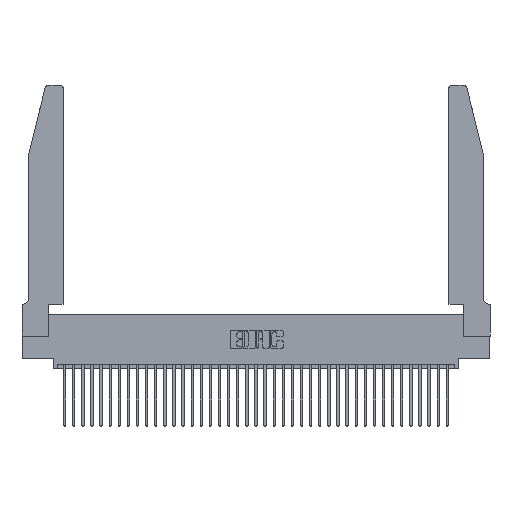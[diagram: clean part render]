
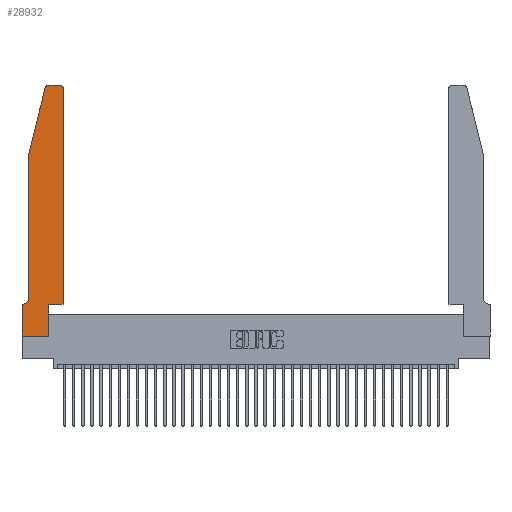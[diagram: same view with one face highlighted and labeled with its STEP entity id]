
A CAD part, top view. The second image highlights one B-rep face of the part: STEP entity #28932.
In plain terms, the highlighted planar face has unit normal (0, 0, 1).
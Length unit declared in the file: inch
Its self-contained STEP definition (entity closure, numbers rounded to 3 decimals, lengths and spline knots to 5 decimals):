
#304 = VERTEX_POINT ( 'NONE', #25919 ) ;
#470 = DIRECTION ( 'NONE',  ( 0., -1., 0. ) ) ;
#1260 = CARTESIAN_POINT ( 'NONE',  ( 0.2605, 2.75, 0.37 ) ) ;
#1505 = EDGE_CURVE ( 'NONE', #33175, #14785, #15760, .T. ) ;
#1660 = DIRECTION ( 'NONE',  ( -1., 0., 0. ) ) ;
#2172 = CARTESIAN_POINT ( 'NONE',  ( 0.4505, 2.72, 0.37 ) ) ;
#2261 = CIRCLE ( 'NONE', #24599, 0.07 ) ;
#3043 = LINE ( 'NONE', #6097, #34599 ) ;
#3149 = ORIENTED_EDGE ( 'NONE', *, *, #13100, .T. ) ;
#3278 = LINE ( 'NONE', #36881, #11348 ) ;
#3804 = CARTESIAN_POINT ( 'NONE',  ( 0.284, 2.72, 0.37 ) ) ;
#3981 = EDGE_CURVE ( 'NONE', #18993, #304, #12584, .T. ) ;
#4358 = DIRECTION ( 'NONE',  ( -1., 0., 0. ) ) ;
#4761 = EDGE_CURVE ( 'NONE', #7552, #15856, #3043, .T. ) ;
#4912 = CARTESIAN_POINT ( 'NONE',  ( 0.0755, 0.42, 0.37 ) ) ;
#4940 = EDGE_CURVE ( 'NONE', #19021, #33175, #29123, .T. ) ;
#5547 = ORIENTED_EDGE ( 'NONE', *, *, #11394, .T. ) ;
#6097 = CARTESIAN_POINT ( 'NONE',  ( 0., 0., 0.37 ) ) ;
#6327 = LINE ( 'NONE', #34366, #13416 ) ;
#6595 = LINE ( 'NONE', #31458, #21521 ) ;
#6859 = DIRECTION ( 'NONE',  ( 1., 0., 0. ) ) ;
#7552 = VERTEX_POINT ( 'NONE', #10192 ) ;
#7788 = AXIS2_PLACEMENT_3D ( 'NONE', #24036, #35851, #18290 ) ;
#7964 = CARTESIAN_POINT ( 'NONE',  ( 0.25487, 2.72718, 0.37 ) ) ;
#8572 = VERTEX_POINT ( 'NONE', #38523 ) ;
#9443 = CARTESIAN_POINT ( 'NONE',  ( 0.4505, 0.35, 0.37 ) ) ;
#10177 = DIRECTION ( 'NONE',  ( 1., 0., 0. ) ) ;
#10192 = CARTESIAN_POINT ( 'NONE',  ( 0., 0.35, 0.37 ) ) ;
#10403 = VECTOR ( 'NONE', #24217, 39.37008 ) ;
#11271 = ORIENTED_EDGE ( 'NONE', *, *, #35568, .T. ) ;
#11348 = VECTOR ( 'NONE', #13345, 39.37008 ) ;
#11394 = EDGE_CURVE ( 'NONE', #8572, #18993, #33924, .T. ) ;
#11658 = ORIENTED_EDGE ( 'NONE', *, *, #33771, .T. ) ;
#12418 = FACE_OUTER_BOUND ( 'NONE', #30253, .T. ) ;
#12584 = CIRCLE ( 'NONE', #25155, 0.03 ) ;
#13100 = EDGE_CURVE ( 'NONE', #26247, #27974, #2261, .T. ) ;
#13345 = DIRECTION ( 'NONE',  ( -1., 0., 0. ) ) ;
#13416 = VECTOR ( 'NONE', #28503, 39.37008 ) ;
#13908 = VECTOR ( 'NONE', #35479, 39.37008 ) ;
#14070 = ORIENTED_EDGE ( 'NONE', *, *, #4940, .T. ) ;
#14584 = CARTESIAN_POINT ( 'NONE',  ( 0.4205, 2.72, 0.37 ) ) ;
#14785 = VERTEX_POINT ( 'NONE', #27645 ) ;
#15078 = AXIS2_PLACEMENT_3D ( 'NONE', #3804, #24675, #6859 ) ;
#15760 = LINE ( 'NONE', #38482, #13908 ) ;
#15856 = VERTEX_POINT ( 'NONE', #31066 ) ;
#15868 = VECTOR ( 'NONE', #470, 39.37008 ) ;
#16857 = DIRECTION ( 'NONE',  ( 1., 0., 0. ) ) ;
#17361 = CARTESIAN_POINT ( 'NONE',  ( 0.284, 2.75, 0.37 ) ) ;
#17573 = DIRECTION ( 'NONE',  ( 1., 0., 0. ) ) ;
#18290 = DIRECTION ( 'NONE',  ( 1., 0., 0. ) ) ;
#18993 = VERTEX_POINT ( 'NONE', #2172 ) ;
#19021 = VERTEX_POINT ( 'NONE', #17361 ) ;
#19700 = DIRECTION ( 'NONE',  ( 0., 0., -1. ) ) ;
#20292 = VERTEX_POINT ( 'NONE', #37680 ) ;
#20692 = VECTOR ( 'NONE', #10177, 39.37008 ) ;
#21521 = VECTOR ( 'NONE', #16857, 39.37008 ) ;
#22002 = CARTESIAN_POINT ( 'NONE',  ( 0., 0., 0.37 ) ) ;
#22232 = ORIENTED_EDGE ( 'NONE', *, *, #3981, .T. ) ;
#22586 = ORIENTED_EDGE ( 'NONE', *, *, #33668, .T. ) ;
#23254 = EDGE_CURVE ( 'NONE', #15856, #20292, #28497, .T. ) ;
#23681 = LINE ( 'NONE', #33263, #15868 ) ;
#23896 = DIRECTION ( 'NONE',  ( 0., -1., 0. ) ) ;
#24036 = CARTESIAN_POINT ( 'NONE',  ( 0., 0.35, 0.37 ) ) ;
#24217 = DIRECTION ( 'NONE',  ( 0., 1., 0. ) ) ;
#24599 = AXIS2_PLACEMENT_3D ( 'NONE', #37275, #19700, #1660 ) ;
#24671 = VECTOR ( 'NONE', #4358, 39.37008 ) ;
#24675 = DIRECTION ( 'NONE',  ( 0., 0., 1. ) ) ;
#25155 = AXIS2_PLACEMENT_3D ( 'NONE', #14584, #35128, #17573 ) ;
#25919 = CARTESIAN_POINT ( 'NONE',  ( 0.4205, 2.75, 0.37 ) ) ;
#26247 = VERTEX_POINT ( 'NONE', #4912 ) ;
#27224 = ORIENTED_EDGE ( 'NONE', *, *, #23254, .T. ) ;
#27645 = CARTESIAN_POINT ( 'NONE',  ( 0.0755, 2., 0.37 ) ) ;
#27974 = VERTEX_POINT ( 'NONE', #33957 ) ;
#28497 = LINE ( 'NONE', #22002, #20692 ) ;
#28503 = DIRECTION ( 'NONE',  ( 0., 1., 0. ) ) ;
#28932 = ADVANCED_FACE ( 'NONE', ( #12418 ), #32881, .T. ) ;
#29004 = EDGE_CURVE ( 'NONE', #14785, #26247, #23681, .T. ) ;
#29123 = CIRCLE ( 'NONE', #15078, 0.03 ) ;
#30253 = EDGE_LOOP ( 'NONE', ( #11271, #14070, #34969, #38028, #3149, #22586, #33823, #27224, #36115, #11658, #5547, #22232 ) ) ;
#30467 = CARTESIAN_POINT ( 'NONE',  ( 0.2865, 0.35, 0.37 ) ) ;
#31066 = CARTESIAN_POINT ( 'NONE',  ( 0., 0., 0.37 ) ) ;
#31351 = EDGE_CURVE ( 'NONE', #20292, #34916, #6327, .T. ) ;
#31458 = CARTESIAN_POINT ( 'NONE',  ( 0.4505, 0.35, 0.37 ) ) ;
#32881 = PLANE ( 'NONE',  #7788 ) ;
#33175 = VERTEX_POINT ( 'NONE', #7964 ) ;
#33263 = CARTESIAN_POINT ( 'NONE',  ( 0.0755, 2., 0.37 ) ) ;
#33372 = LINE ( 'NONE', #1260, #24671 ) ;
#33668 = EDGE_CURVE ( 'NONE', #27974, #7552, #3278, .T. ) ;
#33771 = EDGE_CURVE ( 'NONE', #34916, #8572, #6595, .T. ) ;
#33823 = ORIENTED_EDGE ( 'NONE', *, *, #4761, .T. ) ;
#33924 = LINE ( 'NONE', #9443, #10403 ) ;
#33957 = CARTESIAN_POINT ( 'NONE',  ( 0.0055, 0.35, 0.37 ) ) ;
#34366 = CARTESIAN_POINT ( 'NONE',  ( 0.2865, 0.35, 0.37 ) ) ;
#34599 = VECTOR ( 'NONE', #23896, 39.37008 ) ;
#34916 = VERTEX_POINT ( 'NONE', #30467 ) ;
#34969 = ORIENTED_EDGE ( 'NONE', *, *, #1505, .T. ) ;
#35128 = DIRECTION ( 'NONE',  ( 0., 0., 1. ) ) ;
#35479 = DIRECTION ( 'NONE',  ( -0.239, -0.971, 0. ) ) ;
#35568 = EDGE_CURVE ( 'NONE', #304, #19021, #33372, .T. ) ;
#35851 = DIRECTION ( 'NONE',  ( 0., 0., 1. ) ) ;
#36115 = ORIENTED_EDGE ( 'NONE', *, *, #31351, .T. ) ;
#36881 = CARTESIAN_POINT ( 'NONE',  ( 0.0755, 0.35, 0.37 ) ) ;
#37275 = CARTESIAN_POINT ( 'NONE',  ( 0.0055, 0.42, 0.37 ) ) ;
#37680 = CARTESIAN_POINT ( 'NONE',  ( 0.2865, 0., 0.37 ) ) ;
#38028 = ORIENTED_EDGE ( 'NONE', *, *, #29004, .T. ) ;
#38482 = CARTESIAN_POINT ( 'NONE',  ( 0.0755, 2., 0.37 ) ) ;
#38523 = CARTESIAN_POINT ( 'NONE',  ( 0.4505, 0.35, 0.37 ) ) ;
